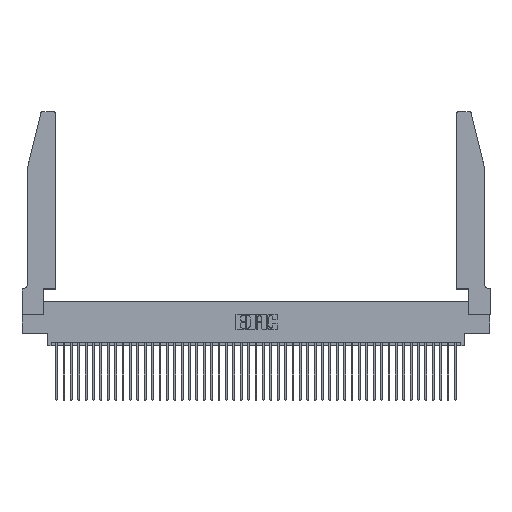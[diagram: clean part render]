
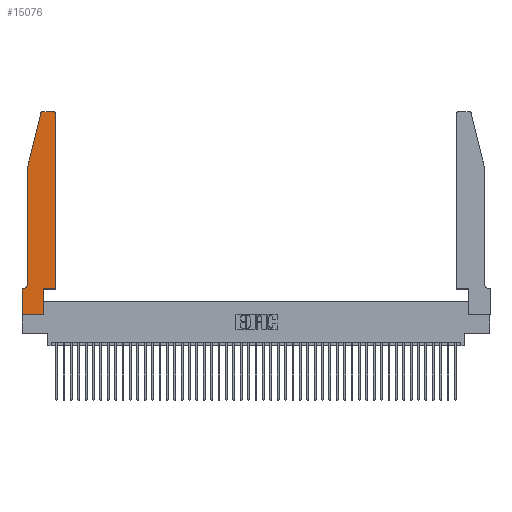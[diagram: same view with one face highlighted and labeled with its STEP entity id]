
A CAD part, top view. The second image highlights one B-rep face of the part: STEP entity #15076.
In plain terms, the highlighted planar face has unit normal (0, 0, 1).
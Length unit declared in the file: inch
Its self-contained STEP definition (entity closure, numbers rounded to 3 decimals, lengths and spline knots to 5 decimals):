
#28 = ORIENTED_EDGE ( 'NONE', *, *, #42005, .T. ) ;
#421 = LINE ( 'NONE', #29383, #18599 ) ;
#731 = AXIS2_PLACEMENT_3D ( 'NONE', #19539, #44323, #23134 ) ;
#1661 = CARTESIAN_POINT ( 'NONE',  ( 0.0755, 2., 0.37 ) ) ;
#1850 = VERTEX_POINT ( 'NONE', #8655 ) ;
#1935 = DIRECTION ( 'NONE',  ( 0., 0., -1. ) ) ;
#1946 = VECTOR ( 'NONE', #14657, 39.37008 ) ;
#2882 = VERTEX_POINT ( 'NONE', #29121 ) ;
#4183 = CARTESIAN_POINT ( 'NONE',  ( 0.0755, 2., 0.37 ) ) ;
#4507 = EDGE_CURVE ( 'NONE', #43041, #2882, #43616, .T. ) ;
#4518 = AXIS2_PLACEMENT_3D ( 'NONE', #28020, #6513, #31577 ) ;
#4859 = VECTOR ( 'NONE', #23906, 39.37008 ) ;
#5010 = PLANE ( 'NONE',  #731 ) ;
#5198 = DIRECTION ( 'NONE',  ( -0.239, -0.971, 0. ) ) ;
#5369 = AXIS2_PLACEMENT_3D ( 'NONE', #15217, #40119, #18880 ) ;
#5384 = EDGE_CURVE ( 'NONE', #1850, #20340, #421, .T. ) ;
#6025 = LINE ( 'NONE', #13027, #4859 ) ;
#6444 = CARTESIAN_POINT ( 'NONE',  ( 0., 0., 0.37 ) ) ;
#6513 = DIRECTION ( 'NONE',  ( 0., 0., 1. ) ) ;
#7700 = AXIS2_PLACEMENT_3D ( 'NONE', #23603, #1935, #27204 ) ;
#7813 = ORIENTED_EDGE ( 'NONE', *, *, #24768, .T. ) ;
#8196 = EDGE_CURVE ( 'NONE', #11077, #19867, #17826, .T. ) ;
#8655 = CARTESIAN_POINT ( 'NONE',  ( 0.0055, 0.35, 0.37 ) ) ;
#8932 = DIRECTION ( 'NONE',  ( -1., 0., 0. ) ) ;
#10245 = EDGE_LOOP ( 'NONE', ( #31803, #18915, #15832, #13560, #40839, #46220, #40143, #7813, #31482, #24772, #30617, #28 ) ) ;
#11077 = VERTEX_POINT ( 'NONE', #22502 ) ;
#11523 = VECTOR ( 'NONE', #8932, 39.37008 ) ;
#12940 = CARTESIAN_POINT ( 'NONE',  ( 0.4205, 2.75, 0.37 ) ) ;
#13027 = CARTESIAN_POINT ( 'NONE',  ( 0.2865, 0.35, 0.37 ) ) ;
#13560 = ORIENTED_EDGE ( 'NONE', *, *, #20568, .T. ) ;
#13660 = CARTESIAN_POINT ( 'NONE',  ( 0., 0.35, 0.37 ) ) ;
#14657 = DIRECTION ( 'NONE',  ( 0., -1., 0. ) ) ;
#14824 = CARTESIAN_POINT ( 'NONE',  ( 0.0755, 2., 0.37 ) ) ;
#15076 = ADVANCED_FACE ( 'NONE', ( #46160 ), #5010, .T. ) ;
#15217 = CARTESIAN_POINT ( 'NONE',  ( 0.284, 2.72, 0.37 ) ) ;
#15832 = ORIENTED_EDGE ( 'NONE', *, *, #8196, .T. ) ;
#15937 = VECTOR ( 'NONE', #45832, 39.37008 ) ;
#16172 = VECTOR ( 'NONE', #25794, 39.37008 ) ;
#17220 = CIRCLE ( 'NONE', #7700, 0.07 ) ;
#17826 = LINE ( 'NONE', #1661, #35626 ) ;
#18599 = VECTOR ( 'NONE', #36454, 39.37008 ) ;
#18880 = DIRECTION ( 'NONE',  ( 1., 0., 0. ) ) ;
#18915 = ORIENTED_EDGE ( 'NONE', *, *, #28047, .T. ) ;
#19474 = VERTEX_POINT ( 'NONE', #12940 ) ;
#19539 = CARTESIAN_POINT ( 'NONE',  ( 0., 0.35, 0.37 ) ) ;
#19867 = VERTEX_POINT ( 'NONE', #14824 ) ;
#20020 = CARTESIAN_POINT ( 'NONE',  ( 0.4505, 2.72, 0.37 ) ) ;
#20340 = VERTEX_POINT ( 'NONE', #13660 ) ;
#20568 = EDGE_CURVE ( 'NONE', #19867, #23928, #21250, .T. ) ;
#21001 = EDGE_CURVE ( 'NONE', #20340, #23401, #24582, .T. ) ;
#21024 = DIRECTION ( 'NONE',  ( 1., 0., 0. ) ) ;
#21071 = CARTESIAN_POINT ( 'NONE',  ( 0.4505, 0.35, 0.37 ) ) ;
#21250 = LINE ( 'NONE', #4183, #16172 ) ;
#21399 = EDGE_CURVE ( 'NONE', #23324, #43041, #6025, .T. ) ;
#22502 = CARTESIAN_POINT ( 'NONE',  ( 0.25487, 2.72718, 0.37 ) ) ;
#23134 = DIRECTION ( 'NONE',  ( 1., 0., 0. ) ) ;
#23246 = EDGE_CURVE ( 'NONE', #23928, #1850, #17220, .T. ) ;
#23324 = VERTEX_POINT ( 'NONE', #27510 ) ;
#23401 = VERTEX_POINT ( 'NONE', #6444 ) ;
#23603 = CARTESIAN_POINT ( 'NONE',  ( 0.0055, 0.42, 0.37 ) ) ;
#23906 = DIRECTION ( 'NONE',  ( 0., 1., 0. ) ) ;
#23928 = VERTEX_POINT ( 'NONE', #24965 ) ;
#24582 = LINE ( 'NONE', #32469, #1946 ) ;
#24768 = EDGE_CURVE ( 'NONE', #23401, #23324, #39860, .T. ) ;
#24772 = ORIENTED_EDGE ( 'NONE', *, *, #4507, .T. ) ;
#24965 = CARTESIAN_POINT ( 'NONE',  ( 0.0755, 0.42, 0.37 ) ) ;
#25794 = DIRECTION ( 'NONE',  ( 0., -1., 0. ) ) ;
#27204 = DIRECTION ( 'NONE',  ( -1., 0., 0. ) ) ;
#27510 = CARTESIAN_POINT ( 'NONE',  ( 0.2865, 0., 0.37 ) ) ;
#28020 = CARTESIAN_POINT ( 'NONE',  ( 0.4205, 2.72, 0.37 ) ) ;
#28047 = EDGE_CURVE ( 'NONE', #45094, #11077, #28594, .T. ) ;
#28485 = CARTESIAN_POINT ( 'NONE',  ( 0.284, 2.75, 0.37 ) ) ;
#28594 = CIRCLE ( 'NONE', #5369, 0.03 ) ;
#29121 = CARTESIAN_POINT ( 'NONE',  ( 0.4505, 0.35, 0.37 ) ) ;
#29383 = CARTESIAN_POINT ( 'NONE',  ( 0.0755, 0.35, 0.37 ) ) ;
#30483 = VECTOR ( 'NONE', #32932, 39.37008 ) ;
#30519 = CARTESIAN_POINT ( 'NONE',  ( 0.2605, 2.75, 0.37 ) ) ;
#30575 = LINE ( 'NONE', #30519, #11523 ) ;
#30617 = ORIENTED_EDGE ( 'NONE', *, *, #35452, .T. ) ;
#31046 = VERTEX_POINT ( 'NONE', #20020 ) ;
#31482 = ORIENTED_EDGE ( 'NONE', *, *, #21399, .T. ) ;
#31577 = DIRECTION ( 'NONE',  ( 1., 0., 0. ) ) ;
#31803 = ORIENTED_EDGE ( 'NONE', *, *, #43783, .T. ) ;
#32469 = CARTESIAN_POINT ( 'NONE',  ( 0., 0., 0.37 ) ) ;
#32629 = CARTESIAN_POINT ( 'NONE',  ( 0., 0., 0.37 ) ) ;
#32932 = DIRECTION ( 'NONE',  ( 1., 0., 0. ) ) ;
#34225 = VECTOR ( 'NONE', #21024, 39.37008 ) ;
#35452 = EDGE_CURVE ( 'NONE', #2882, #31046, #43211, .T. ) ;
#35626 = VECTOR ( 'NONE', #5198, 39.37008 ) ;
#36454 = DIRECTION ( 'NONE',  ( -1., 0., 0. ) ) ;
#39503 = CIRCLE ( 'NONE', #4518, 0.03 ) ;
#39860 = LINE ( 'NONE', #32629, #30483 ) ;
#40119 = DIRECTION ( 'NONE',  ( 0., 0., 1. ) ) ;
#40143 = ORIENTED_EDGE ( 'NONE', *, *, #21001, .T. ) ;
#40839 = ORIENTED_EDGE ( 'NONE', *, *, #23246, .T. ) ;
#42005 = EDGE_CURVE ( 'NONE', #31046, #19474, #39503, .T. ) ;
#42080 = CARTESIAN_POINT ( 'NONE',  ( 0.4505, 0.35, 0.37 ) ) ;
#43041 = VERTEX_POINT ( 'NONE', #43525 ) ;
#43211 = LINE ( 'NONE', #21071, #15937 ) ;
#43525 = CARTESIAN_POINT ( 'NONE',  ( 0.2865, 0.35, 0.37 ) ) ;
#43616 = LINE ( 'NONE', #42080, #34225 ) ;
#43783 = EDGE_CURVE ( 'NONE', #19474, #45094, #30575, .T. ) ;
#44323 = DIRECTION ( 'NONE',  ( 0., 0., 1. ) ) ;
#45094 = VERTEX_POINT ( 'NONE', #28485 ) ;
#45832 = DIRECTION ( 'NONE',  ( 0., 1., 0. ) ) ;
#46160 = FACE_OUTER_BOUND ( 'NONE', #10245, .T. ) ;
#46220 = ORIENTED_EDGE ( 'NONE', *, *, #5384, .T. ) ;
